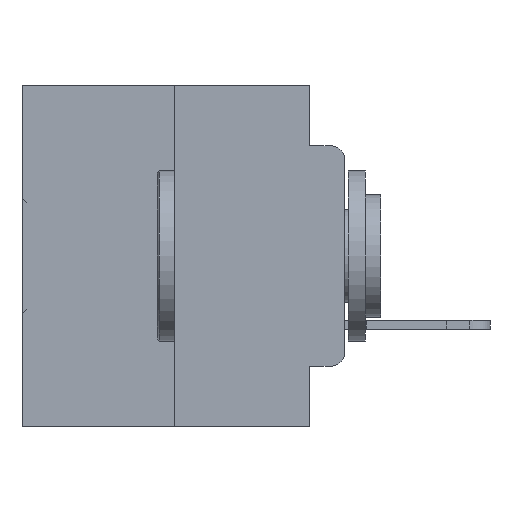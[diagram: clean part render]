
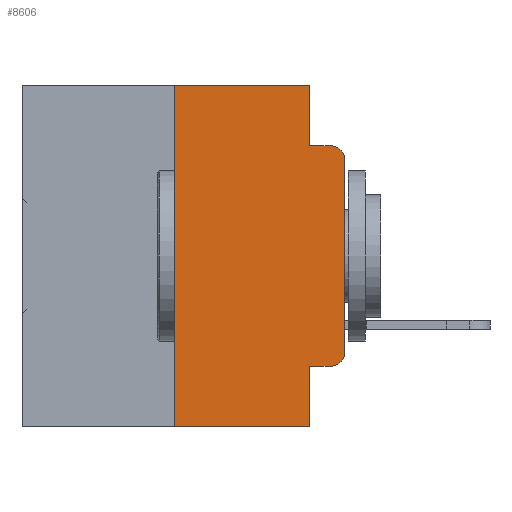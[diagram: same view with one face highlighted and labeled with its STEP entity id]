
A CAD part, left-side view. The second image highlights one B-rep face of the part: STEP entity #8606.
In plain terms, the highlighted planar face has unit normal (-1, 0, 0).
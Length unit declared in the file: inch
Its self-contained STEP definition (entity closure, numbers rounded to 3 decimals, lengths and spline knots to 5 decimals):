
#220 = DIRECTION ( 'NONE',  ( 0., 0., 1. ) ) ;
#346 = DIRECTION ( 'NONE',  ( -1., 0., 0. ) ) ;
#751 = ORIENTED_EDGE ( 'NONE', *, *, #18212, .T. ) ;
#805 = CARTESIAN_POINT ( 'NONE',  ( 0., 0.25, -0.5 ) ) ;
#936 = ORIENTED_EDGE ( 'NONE', *, *, #11887, .F. ) ;
#1658 = CARTESIAN_POINT ( 'NONE',  ( 0., 0., -0.3915 ) ) ;
#2469 = CARTESIAN_POINT ( 'NONE',  ( 0., 0.051, 0. ) ) ;
#2966 = VECTOR ( 'NONE', #30496, 39.37008 ) ;
#3913 = CARTESIAN_POINT ( 'NONE',  ( 0., 0.473, 0. ) ) ;
#4265 = DIRECTION ( 'NONE',  ( 0., -1., 0. ) ) ;
#4772 = CIRCLE ( 'NONE', #24484, 0.02 ) ;
#5403 = VERTEX_POINT ( 'NONE', #24035 ) ;
#6118 = VERTEX_POINT ( 'NONE', #23958 ) ;
#6641 = CARTESIAN_POINT ( 'NONE',  ( 0., 0.25, 0. ) ) ;
#6817 = CARTESIAN_POINT ( 'NONE',  ( 0., 0.051, -0.5 ) ) ;
#7454 = CARTESIAN_POINT ( 'NONE',  ( 0., 0.02, -0.4115 ) ) ;
#7899 = LINE ( 'NONE', #6641, #16314 ) ;
#8606 = ADVANCED_FACE ( 'NONE', ( #29815 ), #24038, .F. ) ;
#8905 = LINE ( 'NONE', #31182, #15534 ) ;
#8926 = EDGE_LOOP ( 'NONE', ( #23167, #15283, #14968, #19923, #936, #11731, #20906, #20007, #12680, #751 ) ) ;
#9399 = CARTESIAN_POINT ( 'NONE',  ( 0., 0.051, 0. ) ) ;
#10589 = VECTOR ( 'NONE', #30689, 39.37008 ) ;
#11731 = ORIENTED_EDGE ( 'NONE', *, *, #18107, .F. ) ;
#11887 = EDGE_CURVE ( 'NONE', #6118, #24820, #19419, .T. ) ;
#11897 = VECTOR ( 'NONE', #4265, 39.37008 ) ;
#12021 = CARTESIAN_POINT ( 'NONE',  ( 0., 0.051, -0.0885 ) ) ;
#12680 = ORIENTED_EDGE ( 'NONE', *, *, #18202, .T. ) ;
#12946 = DIRECTION ( 'NONE',  ( 0., -1., 0. ) ) ;
#14968 = ORIENTED_EDGE ( 'NONE', *, *, #18048, .F. ) ;
#15141 = VERTEX_POINT ( 'NONE', #7454 ) ;
#15283 = ORIENTED_EDGE ( 'NONE', *, *, #18002, .T. ) ;
#15405 = VECTOR ( 'NONE', #23317, 39.37008 ) ;
#15534 = VECTOR ( 'NONE', #12946, 39.37008 ) ;
#15675 = CARTESIAN_POINT ( 'NONE',  ( 0., 0.02, -0.3915 ) ) ;
#16114 = EDGE_CURVE ( 'NONE', #27135, #22467, #8905, .T. ) ;
#16314 = VECTOR ( 'NONE', #25815, 39.37008 ) ;
#17176 = LINE ( 'NONE', #12021, #2966 ) ;
#17431 = CARTESIAN_POINT ( 'NONE',  ( 0., 0.02, -0.1085 ) ) ;
#17997 = EDGE_CURVE ( 'NONE', #28178, #5403, #32392, .T. ) ;
#18002 = EDGE_CURVE ( 'NONE', #5403, #21802, #4772, .T. ) ;
#18048 = EDGE_CURVE ( 'NONE', #30474, #21802, #17176, .T. ) ;
#18100 = EDGE_CURVE ( 'NONE', #24820, #30474, #29369, .T. ) ;
#18107 = EDGE_CURVE ( 'NONE', #27135, #6118, #7899, .T. ) ;
#18113 = EDGE_CURVE ( 'NONE', #28699, #22467, #22715, .T. ) ;
#18202 = EDGE_CURVE ( 'NONE', #28699, #15141, #26213, .T. ) ;
#18212 = EDGE_CURVE ( 'NONE', #15141, #28178, #19438, .T. ) ;
#18548 = DIRECTION ( 'NONE',  ( 0., 0., -1. ) ) ;
#19419 = LINE ( 'NONE', #3913, #20291 ) ;
#19438 = CIRCLE ( 'NONE', #22639, 0.02 ) ;
#19923 = ORIENTED_EDGE ( 'NONE', *, *, #18100, .F. ) ;
#20007 = ORIENTED_EDGE ( 'NONE', *, *, #18113, .F. ) ;
#20291 = VECTOR ( 'NONE', #20915, 39.37008 ) ;
#20310 = DIRECTION ( 'NONE',  ( 0., 0., -1. ) ) ;
#20906 = ORIENTED_EDGE ( 'NONE', *, *, #16114, .T. ) ;
#20915 = DIRECTION ( 'NONE',  ( 0., -1., 0. ) ) ;
#21643 = CARTESIAN_POINT ( 'NONE',  ( 0., 0.02, -0.0885 ) ) ;
#21802 = VERTEX_POINT ( 'NONE', #21643 ) ;
#22467 = VERTEX_POINT ( 'NONE', #6817 ) ;
#22639 = AXIS2_PLACEMENT_3D ( 'NONE', #15675, #33644, #18548 ) ;
#22715 = LINE ( 'NONE', #30784, #15405 ) ;
#22775 = CARTESIAN_POINT ( 'NONE',  ( 0., 0., 0. ) ) ;
#23167 = ORIENTED_EDGE ( 'NONE', *, *, #17997, .T. ) ;
#23317 = DIRECTION ( 'NONE',  ( 0., 0., -1. ) ) ;
#23787 = DIRECTION ( 'NONE',  ( 0., 0., -1. ) ) ;
#23823 = DIRECTION ( 'NONE',  ( 1., 0., 0. ) ) ;
#23958 = CARTESIAN_POINT ( 'NONE',  ( 0., 0.25, 0. ) ) ;
#23961 = CARTESIAN_POINT ( 'NONE',  ( 0., 0.473, 0. ) ) ;
#24035 = CARTESIAN_POINT ( 'NONE',  ( 0., 0., -0.1085 ) ) ;
#24038 = PLANE ( 'NONE',  #29479 ) ;
#24484 = AXIS2_PLACEMENT_3D ( 'NONE', #17431, #346, #20310 ) ;
#24820 = VERTEX_POINT ( 'NONE', #2469 ) ;
#25815 = DIRECTION ( 'NONE',  ( 0., 0., 1. ) ) ;
#25847 = VECTOR ( 'NONE', #220, 39.37008 ) ;
#26020 = CARTESIAN_POINT ( 'NONE',  ( 0., 0.051, -0.4115 ) ) ;
#26213 = LINE ( 'NONE', #31086, #11897 ) ;
#27135 = VERTEX_POINT ( 'NONE', #805 ) ;
#28178 = VERTEX_POINT ( 'NONE', #1658 ) ;
#28699 = VERTEX_POINT ( 'NONE', #26020 ) ;
#29369 = LINE ( 'NONE', #9399, #10589 ) ;
#29479 = AXIS2_PLACEMENT_3D ( 'NONE', #23961, #23823, #23787 ) ;
#29815 = FACE_OUTER_BOUND ( 'NONE', #8926, .T. ) ;
#30474 = VERTEX_POINT ( 'NONE', #33067 ) ;
#30496 = DIRECTION ( 'NONE',  ( 0., -1., 0. ) ) ;
#30689 = DIRECTION ( 'NONE',  ( 0., 0., -1. ) ) ;
#30784 = CARTESIAN_POINT ( 'NONE',  ( 0., 0.051, 0. ) ) ;
#31086 = CARTESIAN_POINT ( 'NONE',  ( 0., 0.051, -0.4115 ) ) ;
#31182 = CARTESIAN_POINT ( 'NONE',  ( 0., 0.473, -0.5 ) ) ;
#32392 = LINE ( 'NONE', #22775, #25847 ) ;
#33067 = CARTESIAN_POINT ( 'NONE',  ( 0., 0.051, -0.0885 ) ) ;
#33644 = DIRECTION ( 'NONE',  ( -1., 0., 0. ) ) ;
